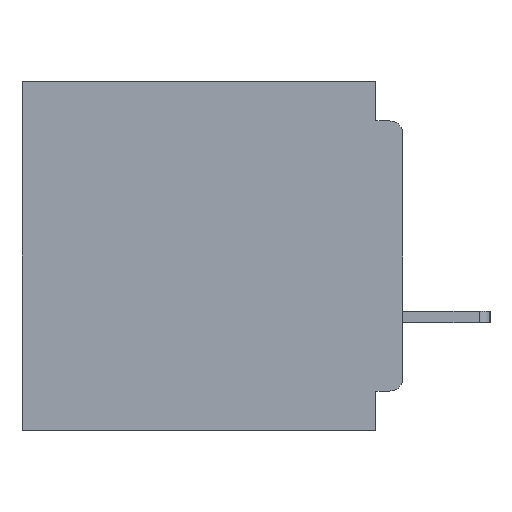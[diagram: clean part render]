
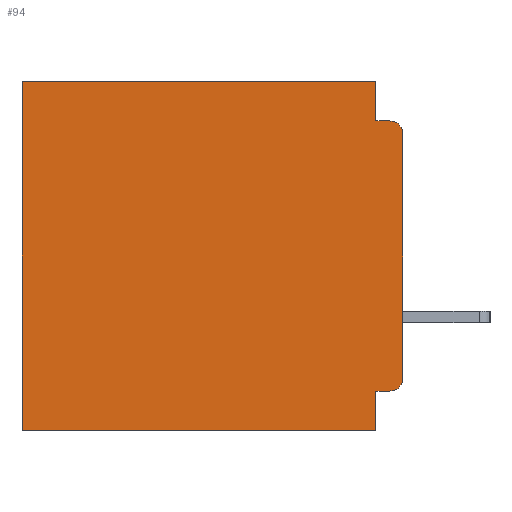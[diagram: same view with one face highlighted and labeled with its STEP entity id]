
A CAD part, left-side view. The second image highlights one B-rep face of the part: STEP entity #94.
In plain terms, the highlighted planar face has unit normal (-1, 0, 0).
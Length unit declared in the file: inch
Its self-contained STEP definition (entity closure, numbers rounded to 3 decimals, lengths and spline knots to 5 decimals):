
#94 = ADVANCED_FACE ( 'NONE', ( #23359 ), #13418, .F. ) ;
#455 = DIRECTION ( 'NONE',  ( 0., -1., 0. ) ) ;
#1212 = VERTEX_POINT ( 'NONE', #12865 ) ;
#1766 = LINE ( 'NONE', #15648, #18769 ) ;
#1982 = EDGE_CURVE ( 'NONE', #15352, #33774, #1766, .T. ) ;
#2418 = LINE ( 'NONE', #34191, #3491 ) ;
#3156 = EDGE_CURVE ( 'NONE', #19810, #25578, #18143, .T. ) ;
#3329 = ORIENTED_EDGE ( 'NONE', *, *, #1982, .F. ) ;
#3491 = VECTOR ( 'NONE', #17158, 39.37008 ) ;
#3754 = CARTESIAN_POINT ( 'NONE',  ( 0.3, 0., -0.045 ) ) ;
#3915 = VERTEX_POINT ( 'NONE', #32565 ) ;
#4553 = VERTEX_POINT ( 'NONE', #36984 ) ;
#5029 = AXIS2_PLACEMENT_3D ( 'NONE', #11528, #14729, #14888 ) ;
#5523 = EDGE_LOOP ( 'NONE', ( #28729, #42920, #38276, #8498, #10633, #37264, #3329, #23546, #15073, #18840 ) ) ;
#5872 = DIRECTION ( 'NONE',  ( 1., 0., 0. ) ) ;
#7163 = CARTESIAN_POINT ( 'NONE',  ( 0.3, 0., -0.4 ) ) ;
#7626 = VECTOR ( 'NONE', #455, 39.37008 ) ;
#8498 = ORIENTED_EDGE ( 'NONE', *, *, #18760, .F. ) ;
#9446 = DIRECTION ( 'NONE',  ( -1., 0., 0. ) ) ;
#9760 = LINE ( 'NONE', #3754, #7626 ) ;
#9979 = EDGE_CURVE ( 'NONE', #34930, #1212, #13069, .T. ) ;
#10236 = CARTESIAN_POINT ( 'NONE',  ( 0.3, 0.031, -0.4 ) ) ;
#10633 = ORIENTED_EDGE ( 'NONE', *, *, #40832, .T. ) ;
#10680 = LINE ( 'NONE', #7163, #18654 ) ;
#11306 = VERTEX_POINT ( 'NONE', #29658 ) ;
#11528 = CARTESIAN_POINT ( 'NONE',  ( 0.3, 0.015, -0.34 ) ) ;
#12285 = DIRECTION ( 'NONE',  ( 0., 1., 0. ) ) ;
#12389 = CARTESIAN_POINT ( 'NONE',  ( 0.3, 0., -0.06 ) ) ;
#12865 = CARTESIAN_POINT ( 'NONE',  ( 0.3, 0.015, -0.045 ) ) ;
#13069 = CIRCLE ( 'NONE', #39524, 0.015 ) ;
#13418 = PLANE ( 'NONE',  #18314 ) ;
#13489 = CARTESIAN_POINT ( 'NONE',  ( 0.3, 0.015, -0.355 ) ) ;
#14235 = EDGE_CURVE ( 'NONE', #38574, #15352, #2418, .T. ) ;
#14729 = DIRECTION ( 'NONE',  ( -1., 0., 0. ) ) ;
#14888 = DIRECTION ( 'NONE',  ( 0., 0., -1. ) ) ;
#15073 = ORIENTED_EDGE ( 'NONE', *, *, #21378, .F. ) ;
#15352 = VERTEX_POINT ( 'NONE', #10236 ) ;
#15648 = CARTESIAN_POINT ( 'NONE',  ( 0.3, 0., -0.4 ) ) ;
#16692 = VECTOR ( 'NONE', #43330, 39.37008 ) ;
#17158 = DIRECTION ( 'NONE',  ( 0., 0., -1. ) ) ;
#18143 = CIRCLE ( 'NONE', #5029, 0.015 ) ;
#18314 = AXIS2_PLACEMENT_3D ( 'NONE', #21414, #5872, #32495 ) ;
#18654 = VECTOR ( 'NONE', #34451, 39.37008 ) ;
#18760 = EDGE_CURVE ( 'NONE', #11306, #4553, #28160, .T. ) ;
#18769 = VECTOR ( 'NONE', #23898, 39.37008 ) ;
#18840 = ORIENTED_EDGE ( 'NONE', *, *, #3156, .T. ) ;
#19810 = VERTEX_POINT ( 'NONE', #13489 ) ;
#21378 = EDGE_CURVE ( 'NONE', #19810, #38574, #31732, .T. ) ;
#21414 = CARTESIAN_POINT ( 'NONE',  ( 0.3, 0., -0.4 ) ) ;
#22146 = EDGE_CURVE ( 'NONE', #3915, #33774, #25754, .T. ) ;
#22614 = VECTOR ( 'NONE', #25713, 39.37008 ) ;
#23111 = CARTESIAN_POINT ( 'NONE',  ( 0.3, 0.437, -0.4 ) ) ;
#23359 = FACE_OUTER_BOUND ( 'NONE', #5523, .T. ) ;
#23373 = DIRECTION ( 'NONE',  ( 0., 0., -1. ) ) ;
#23546 = ORIENTED_EDGE ( 'NONE', *, *, #14235, .F. ) ;
#23898 = DIRECTION ( 'NONE',  ( 0., 1., 0. ) ) ;
#24856 = CARTESIAN_POINT ( 'NONE',  ( 0.3, 0.437, -0.4 ) ) ;
#25104 = EDGE_CURVE ( 'NONE', #34930, #25578, #10680, .T. ) ;
#25578 = VERTEX_POINT ( 'NONE', #27649 ) ;
#25713 = DIRECTION ( 'NONE',  ( 0., 1., 0. ) ) ;
#25754 = LINE ( 'NONE', #23111, #16692 ) ;
#27649 = CARTESIAN_POINT ( 'NONE',  ( 0.3, 0., -0.34 ) ) ;
#28160 = LINE ( 'NONE', #30098, #37171 ) ;
#28729 = ORIENTED_EDGE ( 'NONE', *, *, #25104, .F. ) ;
#29658 = CARTESIAN_POINT ( 'NONE',  ( 0.3, 0.031, 0. ) ) ;
#29854 = CARTESIAN_POINT ( 'NONE',  ( 0.3, 0.015, -0.06 ) ) ;
#30098 = CARTESIAN_POINT ( 'NONE',  ( 0.3, 0.031, 0. ) ) ;
#31732 = LINE ( 'NONE', #42528, #22614 ) ;
#32495 = DIRECTION ( 'NONE',  ( 0., 0., -1. ) ) ;
#32565 = CARTESIAN_POINT ( 'NONE',  ( 0.3, 0.437, 0. ) ) ;
#32717 = CARTESIAN_POINT ( 'NONE',  ( 0.3, 0., 0. ) ) ;
#33296 = DIRECTION ( 'NONE',  ( 0., 0., -1. ) ) ;
#33333 = VECTOR ( 'NONE', #12285, 39.37008 ) ;
#33774 = VERTEX_POINT ( 'NONE', #24856 ) ;
#34191 = CARTESIAN_POINT ( 'NONE',  ( 0.3, 0.031, -0.4 ) ) ;
#34451 = DIRECTION ( 'NONE',  ( 0., 0., -1. ) ) ;
#34930 = VERTEX_POINT ( 'NONE', #12389 ) ;
#36984 = CARTESIAN_POINT ( 'NONE',  ( 0.3, 0.031, -0.045 ) ) ;
#37171 = VECTOR ( 'NONE', #23373, 39.37008 ) ;
#37264 = ORIENTED_EDGE ( 'NONE', *, *, #22146, .T. ) ;
#38276 = ORIENTED_EDGE ( 'NONE', *, *, #41804, .F. ) ;
#38574 = VERTEX_POINT ( 'NONE', #41194 ) ;
#39524 = AXIS2_PLACEMENT_3D ( 'NONE', #29854, #9446, #33296 ) ;
#40832 = EDGE_CURVE ( 'NONE', #11306, #3915, #41173, .T. ) ;
#41173 = LINE ( 'NONE', #32717, #33333 ) ;
#41194 = CARTESIAN_POINT ( 'NONE',  ( 0.3, 0.031, -0.355 ) ) ;
#41804 = EDGE_CURVE ( 'NONE', #4553, #1212, #9760, .T. ) ;
#42528 = CARTESIAN_POINT ( 'NONE',  ( 0.3, 0., -0.355 ) ) ;
#42920 = ORIENTED_EDGE ( 'NONE', *, *, #9979, .T. ) ;
#43330 = DIRECTION ( 'NONE',  ( 0., 0., -1. ) ) ;
